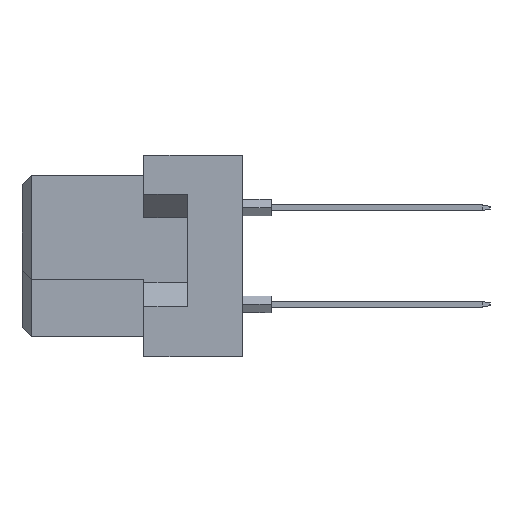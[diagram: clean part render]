
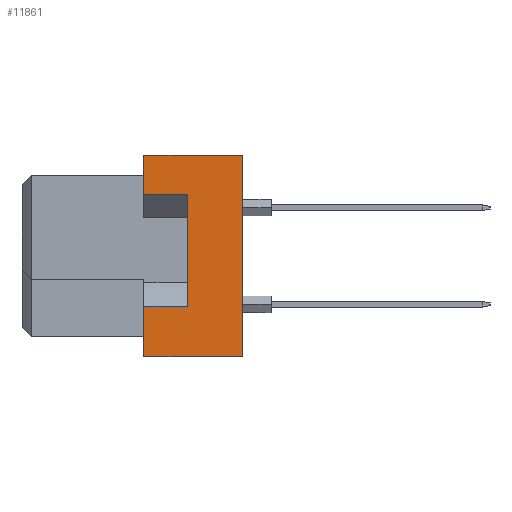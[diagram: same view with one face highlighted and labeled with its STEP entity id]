
A CAD part, left-side view. The second image highlights one B-rep face of the part: STEP entity #11861.
In plain terms, the highlighted planar face has unit normal (-1, 0, 0).
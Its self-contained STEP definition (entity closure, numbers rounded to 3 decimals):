
#1070 = ORIENTED_EDGE ( 'NONE', *, *, #30091, .T. ) ;
#1282 = CARTESIAN_POINT ( 'NONE',  ( -47.5, -11.6, 5.3 ) ) ;
#1673 = CARTESIAN_POINT ( 'NONE',  ( -47.5, -6.4, 5.3 ) ) ;
#2176 = EDGE_CURVE ( 'NONE', #3508, #12310, #11578, .T. ) ;
#2963 = CARTESIAN_POINT ( 'NONE',  ( -47.5, -11.6, -5.3 ) ) ;
#3508 = VERTEX_POINT ( 'NONE', #32293 ) ;
#3714 = VECTOR ( 'NONE', #34890, 1000. ) ;
#3775 = ORIENTED_EDGE ( 'NONE', *, *, #7509, .T. ) ;
#6254 = CARTESIAN_POINT ( 'NONE',  ( -47.5, -6.4, -5.3 ) ) ;
#7290 = DIRECTION ( 'NONE',  ( 0., 0., 1. ) ) ;
#7509 = EDGE_CURVE ( 'NONE', #17944, #25309, #34278, .T. ) ;
#7892 = CARTESIAN_POINT ( 'NONE',  ( -47.5, -6.4, -5.3 ) ) ;
#9995 = CARTESIAN_POINT ( 'NONE',  ( -47.5, -11.6, 5.3 ) ) ;
#10307 = CARTESIAN_POINT ( 'NONE',  ( -47.5, -8.7, -2.65 ) ) ;
#10677 = ORIENTED_EDGE ( 'NONE', *, *, #27164, .F. ) ;
#11540 = VECTOR ( 'NONE', #7290, 1000. ) ;
#11578 = LINE ( 'NONE', #6254, #34666 ) ;
#11861 = ADVANCED_FACE ( 'NONE', ( #16269 ), #22579, .T. ) ;
#12310 = VERTEX_POINT ( 'NONE', #24912 ) ;
#13258 = CARTESIAN_POINT ( 'NONE',  ( -47.5, -8.7, 3.25 ) ) ;
#14035 = EDGE_CURVE ( 'NONE', #37733, #15019, #25832, .T. ) ;
#14139 = VECTOR ( 'NONE', #17357, 1000. ) ;
#14395 = LINE ( 'NONE', #2963, #38641 ) ;
#14554 = LINE ( 'NONE', #23825, #17309 ) ;
#15019 = VERTEX_POINT ( 'NONE', #1673 ) ;
#15710 = EDGE_LOOP ( 'NONE', ( #18158, #35582, #31666, #3775, #1070, #30660, #10677, #27097 ) ) ;
#15836 = EDGE_CURVE ( 'NONE', #17944, #3508, #14395, .T. ) ;
#15869 = AXIS2_PLACEMENT_3D ( 'NONE', #1282, #37532, #25725 ) ;
#16269 = FACE_OUTER_BOUND ( 'NONE', #15710, .T. ) ;
#17309 = VECTOR ( 'NONE', #21259, 1000. ) ;
#17357 = DIRECTION ( 'NONE',  ( 0., 0., 1. ) ) ;
#17492 = DIRECTION ( 'NONE',  ( 0., 0., 1. ) ) ;
#17944 = VERTEX_POINT ( 'NONE', #35949 ) ;
#18019 = CARTESIAN_POINT ( 'NONE',  ( -47.5, -8.7, -2.65 ) ) ;
#18158 = ORIENTED_EDGE ( 'NONE', *, *, #21417, .T. ) ;
#20125 = LINE ( 'NONE', #37838, #3714 ) ;
#20179 = LINE ( 'NONE', #34950, #20491 ) ;
#20491 = VECTOR ( 'NONE', #29034, 1000. ) ;
#21259 = DIRECTION ( 'NONE',  ( 0., 1., 0. ) ) ;
#21417 = EDGE_CURVE ( 'NONE', #26066, #12310, #37287, .T. ) ;
#21905 = CARTESIAN_POINT ( 'NONE',  ( -47.5, -6.4, 3.25 ) ) ;
#22579 = PLANE ( 'NONE',  #15869 ) ;
#23825 = CARTESIAN_POINT ( 'NONE',  ( -47.5, -8.7, 3.25 ) ) ;
#24912 = CARTESIAN_POINT ( 'NONE',  ( -47.5, -6.4, -2.65 ) ) ;
#25309 = VERTEX_POINT ( 'NONE', #9995 ) ;
#25725 = DIRECTION ( 'NONE',  ( 0., 0., 1. ) ) ;
#25832 = LINE ( 'NONE', #7892, #14139 ) ;
#26066 = VERTEX_POINT ( 'NONE', #18019 ) ;
#26402 = DIRECTION ( 'NONE',  ( 0., 1., 0. ) ) ;
#27097 = ORIENTED_EDGE ( 'NONE', *, *, #30750, .F. ) ;
#27164 = EDGE_CURVE ( 'NONE', #37323, #37733, #14554, .T. ) ;
#29034 = DIRECTION ( 'NONE',  ( 0., 1., 0. ) ) ;
#30091 = EDGE_CURVE ( 'NONE', #25309, #15019, #20179, .T. ) ;
#30660 = ORIENTED_EDGE ( 'NONE', *, *, #14035, .F. ) ;
#30750 = EDGE_CURVE ( 'NONE', #26066, #37323, #20125, .T. ) ;
#31666 = ORIENTED_EDGE ( 'NONE', *, *, #15836, .F. ) ;
#32293 = CARTESIAN_POINT ( 'NONE',  ( -47.5, -6.4, -5.3 ) ) ;
#34149 = DIRECTION ( 'NONE',  ( 0., 1., 0. ) ) ;
#34278 = LINE ( 'NONE', #37040, #11540 ) ;
#34666 = VECTOR ( 'NONE', #17492, 1000. ) ;
#34890 = DIRECTION ( 'NONE',  ( 0., 0., 1. ) ) ;
#34950 = CARTESIAN_POINT ( 'NONE',  ( -47.5, -11.6, 5.3 ) ) ;
#35582 = ORIENTED_EDGE ( 'NONE', *, *, #2176, .F. ) ;
#35687 = VECTOR ( 'NONE', #34149, 1000. ) ;
#35949 = CARTESIAN_POINT ( 'NONE',  ( -47.5, -11.6, -5.3 ) ) ;
#37040 = CARTESIAN_POINT ( 'NONE',  ( -47.5, -11.6, 5.3 ) ) ;
#37287 = LINE ( 'NONE', #10307, #35687 ) ;
#37323 = VERTEX_POINT ( 'NONE', #13258 ) ;
#37532 = DIRECTION ( 'NONE',  ( -1., 0., 0. ) ) ;
#37733 = VERTEX_POINT ( 'NONE', #21905 ) ;
#37838 = CARTESIAN_POINT ( 'NONE',  ( -47.5, -8.7, -2.65 ) ) ;
#38641 = VECTOR ( 'NONE', #26402, 1000. ) ;
